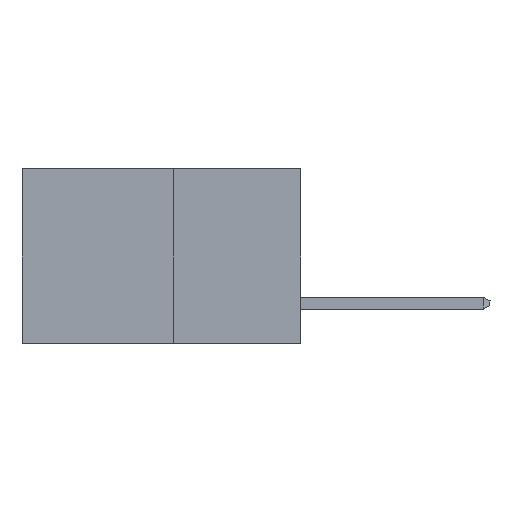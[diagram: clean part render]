
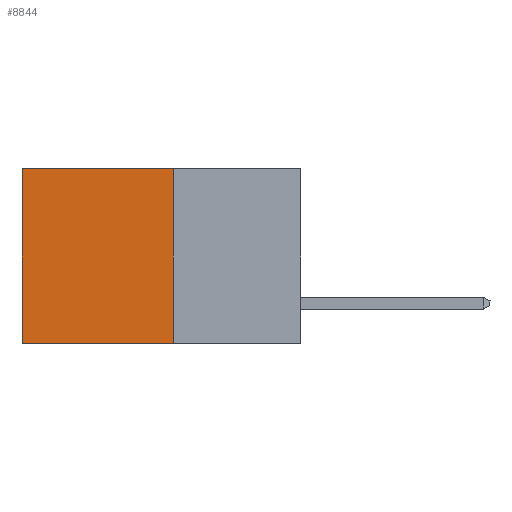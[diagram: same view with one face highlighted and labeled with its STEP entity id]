
A CAD part, left-side view. The second image highlights one B-rep face of the part: STEP entity #8844.
In plain terms, the highlighted planar face has unit normal (-1, 0, 0).
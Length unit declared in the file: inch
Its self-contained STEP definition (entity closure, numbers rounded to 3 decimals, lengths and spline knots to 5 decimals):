
#540 = VECTOR ( 'NONE', #9585, 39.37008 ) ;
#843 = CARTESIAN_POINT ( 'NONE',  ( 0.277, 0.27, -0.37 ) ) ;
#1044 = DIRECTION ( 'NONE',  ( 0., 0., -1. ) ) ;
#1136 = AXIS2_PLACEMENT_3D ( 'NONE', #8144, #3432, #8902 ) ;
#1180 = LINE ( 'NONE', #5108, #7802 ) ;
#1334 = ORIENTED_EDGE ( 'NONE', *, *, #5356, .F. ) ;
#1477 = DIRECTION ( 'NONE',  ( 0., 0., -1. ) ) ;
#1505 = ORIENTED_EDGE ( 'NONE', *, *, #6299, .T. ) ;
#2176 = EDGE_CURVE ( 'NONE', #7647, #2242, #9216, .T. ) ;
#2184 = LINE ( 'NONE', #2274, #8499 ) ;
#2242 = VERTEX_POINT ( 'NONE', #8834 ) ;
#2274 = CARTESIAN_POINT ( 'NONE',  ( 0.277, 0.27, -0.37 ) ) ;
#2698 = EDGE_LOOP ( 'NONE', ( #1505, #5199, #1334, #10180 ) ) ;
#3432 = DIRECTION ( 'NONE',  ( 1., 0., 0. ) ) ;
#4693 = CARTESIAN_POINT ( 'NONE',  ( 0.277, 0.27, -0.37 ) ) ;
#4870 = LINE ( 'NONE', #843, #8992 ) ;
#5108 = CARTESIAN_POINT ( 'NONE',  ( 0.277, 0.59, -0.37 ) ) ;
#5199 = ORIENTED_EDGE ( 'NONE', *, *, #6103, .F. ) ;
#5337 = VERTEX_POINT ( 'NONE', #4693 ) ;
#5356 = EDGE_CURVE ( 'NONE', #7647, #5337, #2184, .T. ) ;
#5381 = VERTEX_POINT ( 'NONE', #6337 ) ;
#5606 = CARTESIAN_POINT ( 'NONE',  ( 0.277, 0.27, 0. ) ) ;
#5827 = PLANE ( 'NONE',  #1136 ) ;
#6103 = EDGE_CURVE ( 'NONE', #5337, #5381, #4870, .T. ) ;
#6299 = EDGE_CURVE ( 'NONE', #2242, #5381, #1180, .T. ) ;
#6337 = CARTESIAN_POINT ( 'NONE',  ( 0.277, 0.59, -0.37 ) ) ;
#6488 = DIRECTION ( 'NONE',  ( 0., 1., 0. ) ) ;
#7257 = FACE_OUTER_BOUND ( 'NONE', #2698, .T. ) ;
#7647 = VERTEX_POINT ( 'NONE', #9739 ) ;
#7802 = VECTOR ( 'NONE', #1044, 39.37008 ) ;
#8144 = CARTESIAN_POINT ( 'NONE',  ( 0.277, 0.27, -0.37 ) ) ;
#8499 = VECTOR ( 'NONE', #1477, 39.37008 ) ;
#8834 = CARTESIAN_POINT ( 'NONE',  ( 0.277, 0.59, 0. ) ) ;
#8844 = ADVANCED_FACE ( 'NONE', ( #7257 ), #5827, .F. ) ;
#8902 = DIRECTION ( 'NONE',  ( 0., 0., -1. ) ) ;
#8992 = VECTOR ( 'NONE', #6488, 39.37008 ) ;
#9216 = LINE ( 'NONE', #5606, #540 ) ;
#9585 = DIRECTION ( 'NONE',  ( 0., 1., 0. ) ) ;
#9739 = CARTESIAN_POINT ( 'NONE',  ( 0.277, 0.27, 0. ) ) ;
#10180 = ORIENTED_EDGE ( 'NONE', *, *, #2176, .T. ) ;
